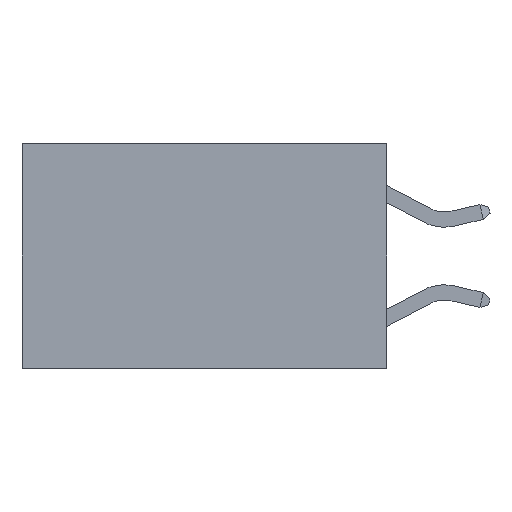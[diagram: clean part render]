
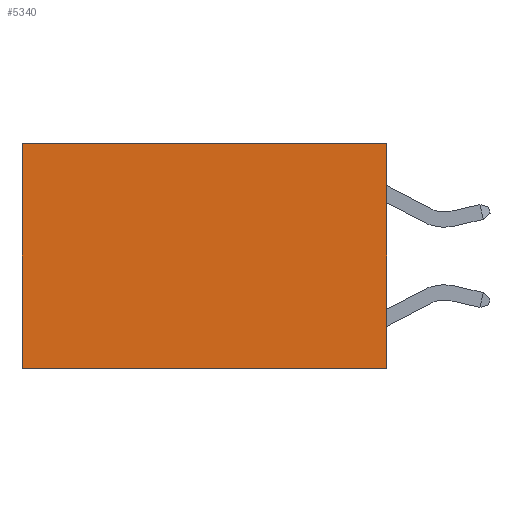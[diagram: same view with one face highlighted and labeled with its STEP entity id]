
A CAD part, left-side view. The second image highlights one B-rep face of the part: STEP entity #5340.
In plain terms, the highlighted planar face has unit normal (-1, 0, 0).
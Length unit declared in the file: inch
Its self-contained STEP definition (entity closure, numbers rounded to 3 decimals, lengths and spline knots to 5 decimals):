
#123 = CARTESIAN_POINT ( 'NONE',  ( 0.2625, 0., -0.37 ) ) ;
#731 = LINE ( 'NONE', #6069, #1983 ) ;
#851 = LINE ( 'NONE', #123, #3953 ) ;
#927 = ORIENTED_EDGE ( 'NONE', *, *, #2533, .F. ) ;
#1229 = CARTESIAN_POINT ( 'NONE',  ( 0.2625, 0., -0.37 ) ) ;
#1416 = EDGE_CURVE ( 'NONE', #9294, #9053, #851, .T. ) ;
#1549 = CARTESIAN_POINT ( 'NONE',  ( 0.2625, 0.6, -0.37 ) ) ;
#1581 = AXIS2_PLACEMENT_3D ( 'NONE', #6082, #7616, #9269 ) ;
#1662 = DIRECTION ( 'NONE',  ( 0., 1., 0. ) ) ;
#1876 = CARTESIAN_POINT ( 'NONE',  ( 0.2625, 0.6, 0. ) ) ;
#1983 = VECTOR ( 'NONE', #1662, 39.37008 ) ;
#2319 = DIRECTION ( 'NONE',  ( 0., 1., 0. ) ) ;
#2523 = DIRECTION ( 'NONE',  ( 0., 0., -1. ) ) ;
#2533 = EDGE_CURVE ( 'NONE', #7917, #9294, #5471, .T. ) ;
#2646 = CARTESIAN_POINT ( 'NONE',  ( 0.2625, 0.6, 0. ) ) ;
#3265 = CARTESIAN_POINT ( 'NONE',  ( 0.2625, 0., 0. ) ) ;
#3293 = PLANE ( 'NONE',  #1581 ) ;
#3345 = CARTESIAN_POINT ( 'NONE',  ( 0.2625, 0., 0. ) ) ;
#3435 = LINE ( 'NONE', #2646, #8701 ) ;
#3574 = EDGE_CURVE ( 'NONE', #7917, #4882, #731, .T. ) ;
#3695 = ORIENTED_EDGE ( 'NONE', *, *, #8286, .T. ) ;
#3953 = VECTOR ( 'NONE', #2319, 39.37008 ) ;
#4882 = VERTEX_POINT ( 'NONE', #1876 ) ;
#5340 = ADVANCED_FACE ( 'NONE', ( #6941 ), #3293, .F. ) ;
#5418 = ORIENTED_EDGE ( 'NONE', *, *, #1416, .F. ) ;
#5471 = LINE ( 'NONE', #3265, #5755 ) ;
#5755 = VECTOR ( 'NONE', #2523, 39.37008 ) ;
#6069 = CARTESIAN_POINT ( 'NONE',  ( 0.2625, 0., 0. ) ) ;
#6082 = CARTESIAN_POINT ( 'NONE',  ( 0.2625, 0., 0. ) ) ;
#6577 = EDGE_LOOP ( 'NONE', ( #3695, #5418, #927, #8235 ) ) ;
#6941 = FACE_OUTER_BOUND ( 'NONE', #6577, .T. ) ;
#7616 = DIRECTION ( 'NONE',  ( 1., 0., 0. ) ) ;
#7917 = VERTEX_POINT ( 'NONE', #3345 ) ;
#8235 = ORIENTED_EDGE ( 'NONE', *, *, #3574, .T. ) ;
#8286 = EDGE_CURVE ( 'NONE', #4882, #9053, #3435, .T. ) ;
#8568 = DIRECTION ( 'NONE',  ( 0., 0., -1. ) ) ;
#8701 = VECTOR ( 'NONE', #8568, 39.37008 ) ;
#9053 = VERTEX_POINT ( 'NONE', #1549 ) ;
#9269 = DIRECTION ( 'NONE',  ( 0., 0., -1. ) ) ;
#9294 = VERTEX_POINT ( 'NONE', #1229 ) ;
